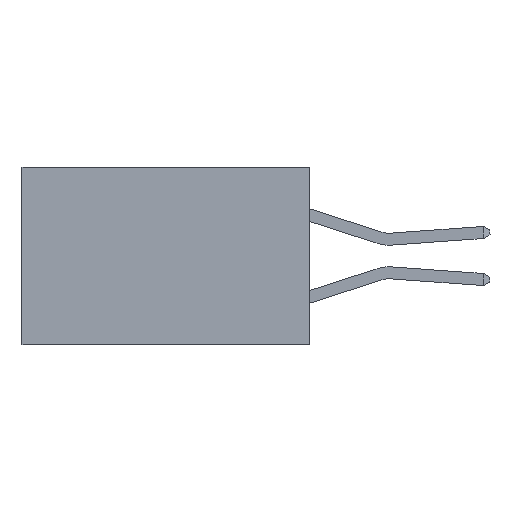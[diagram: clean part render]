
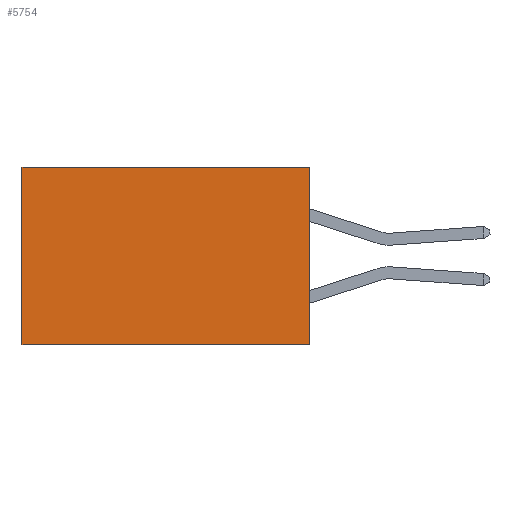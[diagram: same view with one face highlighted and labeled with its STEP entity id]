
A CAD part, left-side view. The second image highlights one B-rep face of the part: STEP entity #5754.
In plain terms, the highlighted planar face has unit normal (-1, 0, 0).
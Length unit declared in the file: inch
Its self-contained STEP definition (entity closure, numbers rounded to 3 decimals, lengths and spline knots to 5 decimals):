
#221 = VERTEX_POINT ( 'NONE', #12800 ) ;
#1982 = ORIENTED_EDGE ( 'NONE', *, *, #3027, .T. ) ;
#2297 = VERTEX_POINT ( 'NONE', #5884 ) ;
#2734 = LINE ( 'NONE', #10227, #13624 ) ;
#3027 = EDGE_CURVE ( 'NONE', #2297, #3550, #2734, .T. ) ;
#3040 = CARTESIAN_POINT ( 'NONE',  ( 0.298, 0., -0.37 ) ) ;
#3550 = VERTEX_POINT ( 'NONE', #11583 ) ;
#3928 = VECTOR ( 'NONE', #11820, 39.37008 ) ;
#4107 = LINE ( 'NONE', #4817, #6777 ) ;
#4604 = LINE ( 'NONE', #9081, #3928 ) ;
#4817 = CARTESIAN_POINT ( 'NONE',  ( 0.298, 0., 0. ) ) ;
#5040 = PLANE ( 'NONE',  #11864 ) ;
#5052 = LINE ( 'NONE', #8793, #10803 ) ;
#5184 = EDGE_CURVE ( 'NONE', #9348, #3550, #5052, .T. ) ;
#5754 = ADVANCED_FACE ( 'NONE', ( #6993 ), #5040, .F. ) ;
#5884 = CARTESIAN_POINT ( 'NONE',  ( 0.298, 0.6, 0. ) ) ;
#6777 = VECTOR ( 'NONE', #10284, 39.37008 ) ;
#6993 = FACE_OUTER_BOUND ( 'NONE', #11169, .T. ) ;
#8125 = EDGE_CURVE ( 'NONE', #221, #2297, #4604, .T. ) ;
#8359 = ORIENTED_EDGE ( 'NONE', *, *, #5184, .F. ) ;
#8462 = DIRECTION ( 'NONE',  ( 0., 1., 0. ) ) ;
#8793 = CARTESIAN_POINT ( 'NONE',  ( 0.298, 0., -0.37 ) ) ;
#8923 = ORIENTED_EDGE ( 'NONE', *, *, #8125, .T. ) ;
#9081 = CARTESIAN_POINT ( 'NONE',  ( 0.298, 0., 0. ) ) ;
#9239 = ORIENTED_EDGE ( 'NONE', *, *, #10886, .F. ) ;
#9348 = VERTEX_POINT ( 'NONE', #3040 ) ;
#10155 = DIRECTION ( 'NONE',  ( 0., 0., -1. ) ) ;
#10227 = CARTESIAN_POINT ( 'NONE',  ( 0.298, 0.6, 0. ) ) ;
#10284 = DIRECTION ( 'NONE',  ( 0., 0., -1. ) ) ;
#10490 = DIRECTION ( 'NONE',  ( 0., 0., -1. ) ) ;
#10803 = VECTOR ( 'NONE', #8462, 39.37008 ) ;
#10831 = CARTESIAN_POINT ( 'NONE',  ( 0.298, 0., 0. ) ) ;
#10886 = EDGE_CURVE ( 'NONE', #221, #9348, #4107, .T. ) ;
#11169 = EDGE_LOOP ( 'NONE', ( #1982, #8359, #9239, #8923 ) ) ;
#11583 = CARTESIAN_POINT ( 'NONE',  ( 0.298, 0.6, -0.37 ) ) ;
#11634 = DIRECTION ( 'NONE',  ( 1., 0., 0. ) ) ;
#11820 = DIRECTION ( 'NONE',  ( 0., 1., 0. ) ) ;
#11864 = AXIS2_PLACEMENT_3D ( 'NONE', #10831, #11634, #10490 ) ;
#12800 = CARTESIAN_POINT ( 'NONE',  ( 0.298, 0., 0. ) ) ;
#13624 = VECTOR ( 'NONE', #10155, 39.37008 ) ;
